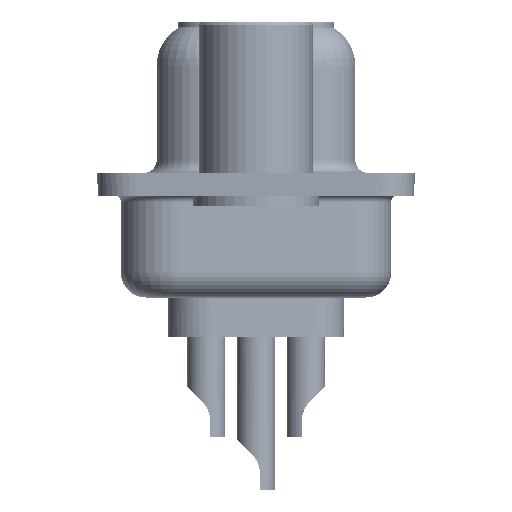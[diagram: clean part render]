
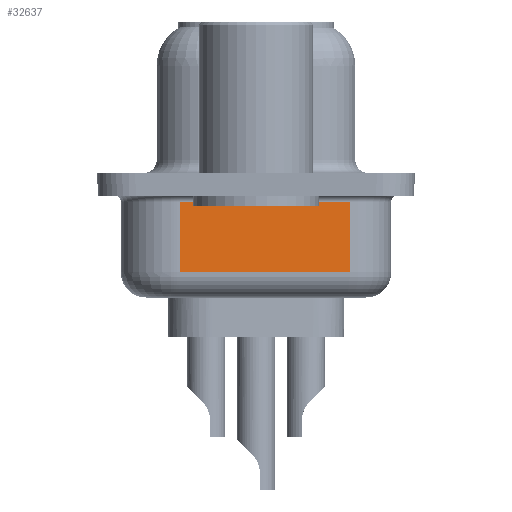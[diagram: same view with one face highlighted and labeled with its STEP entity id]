
A CAD part, left-side view. The second image highlights one B-rep face of the part: STEP entity #32637.
In plain terms, the highlighted planar face has unit normal (-0.985, -0.174, 0).
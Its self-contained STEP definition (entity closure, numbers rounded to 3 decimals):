
#373 = CARTESIAN_POINT ( 'NONE',  ( 3., 3.028, -4.5 ) ) ;
#937 = DIRECTION ( 'NONE',  ( -0.174, 0.985, 0. ) ) ;
#1411 = VERTEX_POINT ( 'NONE', #19484 ) ;
#1870 = LINE ( 'NONE', #14009, #13043 ) ;
#3158 = LINE ( 'NONE', #373, #22558 ) ;
#3778 = VERTEX_POINT ( 'NONE', #34510 ) ;
#5099 = LINE ( 'NONE', #35937, #25233 ) ;
#5923 = ORIENTED_EDGE ( 'NONE', *, *, #17421, .F. ) ;
#6141 = DIRECTION ( 'NONE',  ( 0., 0., 1. ) ) ;
#6351 = PLANE ( 'NONE',  #25054 ) ;
#7837 = DIRECTION ( 'NONE',  ( 0.174, -0.985, 0. ) ) ;
#9061 = CARTESIAN_POINT ( 'NONE',  ( 3., 3.028, -3.5 ) ) ;
#10128 = EDGE_CURVE ( 'NONE', #16161, #1411, #5099, .T. ) ;
#13043 = VECTOR ( 'NONE', #7837, 1000. ) ;
#14009 = CARTESIAN_POINT ( 'NONE',  ( 3., 3.028, -3.5 ) ) ;
#15135 = FACE_OUTER_BOUND ( 'NONE', #32082, .T. ) ;
#16161 = VERTEX_POINT ( 'NONE', #16671 ) ;
#16555 = EDGE_CURVE ( 'NONE', #35484, #3778, #1870, .T. ) ;
#16671 = CARTESIAN_POINT ( 'NONE',  ( 4.191, -3.722, -0.7 ) ) ;
#17379 = ORIENTED_EDGE ( 'NONE', *, *, #16555, .T. ) ;
#17421 = EDGE_CURVE ( 'NONE', #35484, #1411, #3158, .T. ) ;
#17765 = CARTESIAN_POINT ( 'NONE',  ( 3., 3.028, -4.5 ) ) ;
#18400 = DIRECTION ( 'NONE',  ( 0., 0., 1. ) ) ;
#19484 = CARTESIAN_POINT ( 'NONE',  ( 3., 3.028, -0.7 ) ) ;
#22225 = ORIENTED_EDGE ( 'NONE', *, *, #24586, .T. ) ;
#22558 = VECTOR ( 'NONE', #6141, 1000. ) ;
#24190 = LINE ( 'NONE', #30344, #35988 ) ;
#24586 = EDGE_CURVE ( 'NONE', #3778, #16161, #24190, .T. ) ;
#25054 = AXIS2_PLACEMENT_3D ( 'NONE', #17765, #26554, #937 ) ;
#25233 = VECTOR ( 'NONE', #30358, 1000. ) ;
#26554 = DIRECTION ( 'NONE',  ( 0.985, 0.174, 0. ) ) ;
#30344 = CARTESIAN_POINT ( 'NONE',  ( 4.191, -3.722, -4.5 ) ) ;
#30358 = DIRECTION ( 'NONE',  ( -0.174, 0.985, 0. ) ) ;
#32082 = EDGE_LOOP ( 'NONE', ( #5923, #17379, #22225, #32770 ) ) ;
#32637 = ADVANCED_FACE ( 'NONE', ( #15135 ), #6351, .F. ) ;
#32770 = ORIENTED_EDGE ( 'NONE', *, *, #10128, .T. ) ;
#34510 = CARTESIAN_POINT ( 'NONE',  ( 4.191, -3.722, -3.5 ) ) ;
#35484 = VERTEX_POINT ( 'NONE', #9061 ) ;
#35937 = CARTESIAN_POINT ( 'NONE',  ( 3., 3.028, -0.7 ) ) ;
#35988 = VECTOR ( 'NONE', #18400, 1000. ) ;
